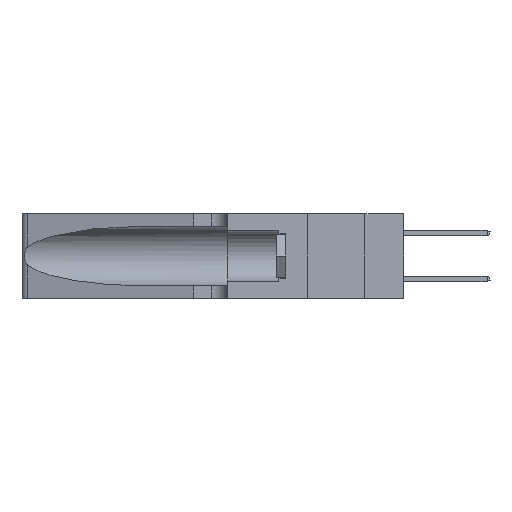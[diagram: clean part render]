
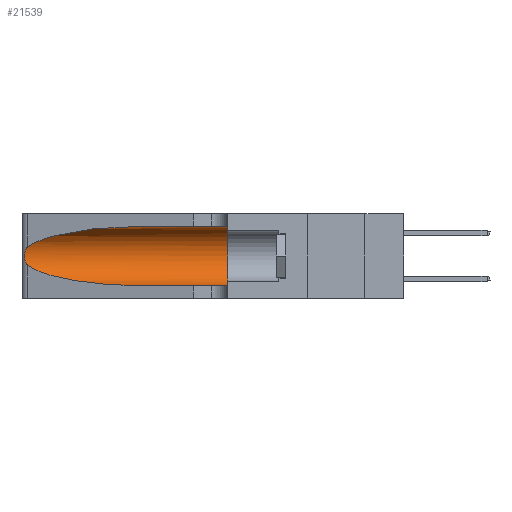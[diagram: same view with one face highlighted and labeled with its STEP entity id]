
A CAD part, left-side view. The second image highlights one B-rep face of the part: STEP entity #21539.
In plain terms, the highlighted cylindrical face has radius 3.308 mm (diameter 6.617 mm), a partial arc.
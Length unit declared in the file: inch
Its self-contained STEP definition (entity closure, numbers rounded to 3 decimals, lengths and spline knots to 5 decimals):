
#81 = ORIENTED_EDGE ( 'NONE', *, *, #700, .T. ) ;
#439 = ORIENTED_EDGE ( 'NONE', *, *, #10689, .T. ) ;
#695 =( BOUNDED_CURVE ( )  B_SPLINE_CURVE ( 3, ( #6078, #23244, #13934, #2161 ),
 .UNSPECIFIED., .F., .T. ) 
 B_SPLINE_CURVE_WITH_KNOTS ( ( 4, 4 ),
 ( 1.5708, 2.84003 ),
 .UNSPECIFIED. ) 
 CURVE ( )  GEOMETRIC_REPRESENTATION_ITEM ( )  RATIONAL_B_SPLINE_CURVE ( ( 1., 0.87, 0.87, 1. ) ) 
 REPRESENTATION_ITEM ( '' )  );
#700 = EDGE_CURVE ( 'NONE', #11478, #8818, #3081, .T. ) ;
#931 = CARTESIAN_POINT ( 'NONE',  ( 0.2373, 1.15595, 0.08982 ) ) ;
#1391 = CARTESIAN_POINT ( 'NONE',  ( 0.25854, 1.2359, 0.20912 ) ) ;
#1404 = ORIENTED_EDGE ( 'NONE', *, *, #21447, .T. ) ;
#1518 = VECTOR ( 'NONE', #3836, 39.37008 ) ;
#1533 = EDGE_CURVE ( 'NONE', #9029, #22695, #22541, .T. ) ;
#2071 = CARTESIAN_POINT ( 'NONE',  ( 0.25487, 1.22718, 0.14631 ) ) ;
#2156 = LINE ( 'NONE', #13624, #1518 ) ;
#2161 = CARTESIAN_POINT ( 'NONE',  ( 0.25487, 1.22718, 0.22369 ) ) ;
#2755 = CARTESIAN_POINT ( 'NONE',  ( 0.1305, 0.72297, 0.31525 ) ) ;
#2770 = VERTEX_POINT ( 'NONE', #15442 ) ;
#3007 = CARTESIAN_POINT ( 'NONE',  ( 0.26075, 1.23896, 0.178 ) ) ;
#3081 = B_SPLINE_CURVE_WITH_KNOTS ( 'NONE', 3,
 ( #7250, #7280, #14345, #20012, #1391, #10024, #15312, #3007, #6337, #12441, #22207, #12812, #7713, #16793 ),
 .UNSPECIFIED., .F., .F.,
 ( 4, 2, 2, 2, 2, 2, 4 ),
 ( 0., 0.00027, 0.00053, 0.00107, 0.0016, 0.00187, 0.00214 ),
 .UNSPECIFIED. ) ;
#3637 = AXIS2_PLACEMENT_3D ( 'NONE', #17673, #8112, #10079 ) ;
#3836 = DIRECTION ( 'NONE',  ( 0., -1., 0. ) ) ;
#3906 = CARTESIAN_POINT ( 'NONE',  ( 0.1305, 1.61858, 0.31525 ) ) ;
#4467 = CARTESIAN_POINT ( 'NONE',  ( 0.25487, 1.22718, 0.22369 ) ) ;
#4722 = ORIENTED_EDGE ( 'NONE', *, *, #1533, .F. ) ;
#5154 = ORIENTED_EDGE ( 'NONE', *, *, #22041, .F. ) ;
#6078 = CARTESIAN_POINT ( 'NONE',  ( 0.1305, 0.72297, 0.31525 ) ) ;
#6337 = CARTESIAN_POINT ( 'NONE',  ( 0.26017, 1.23833, 0.17102 ) ) ;
#6786 = ORIENTED_EDGE ( 'NONE', *, *, #15972, .T. ) ;
#7250 = CARTESIAN_POINT ( 'NONE',  ( 0.25487, 1.22718, 0.22369 ) ) ;
#7280 = CARTESIAN_POINT ( 'NONE',  ( 0.25555, 1.22994, 0.2215 ) ) ;
#7713 = CARTESIAN_POINT ( 'NONE',  ( 0.25555, 1.22993, 0.14849 ) ) ;
#7748 = CARTESIAN_POINT ( 'NONE',  ( 0.1305, 0.35, 0.185 ) ) ;
#8112 = DIRECTION ( 'NONE',  ( 0., -1., 0. ) ) ;
#8818 = VERTEX_POINT ( 'NONE', #2071 ) ;
#8952 = CARTESIAN_POINT ( 'NONE',  ( 0.1305, 0.72297, 0.05475 ) ) ;
#9029 = VERTEX_POINT ( 'NONE', #2755 ) ;
#9606 = FACE_OUTER_BOUND ( 'NONE', #15611, .T. ) ;
#9713 = DIRECTION ( 'NONE',  ( 0., 0., 1. ) ) ;
#10024 = CARTESIAN_POINT ( 'NONE',  ( 0.26018, 1.23835, 0.19895 ) ) ;
#10077 =( BOUNDED_CURVE ( )  B_SPLINE_CURVE ( 3, ( #18459, #931, #20355, #8952 ),
 .UNSPECIFIED., .F., .T. ) 
 B_SPLINE_CURVE_WITH_KNOTS ( ( 4, 4 ),
 ( 3.44316, 4.71239 ),
 .UNSPECIFIED. ) 
 CURVE ( )  GEOMETRIC_REPRESENTATION_ITEM ( )  RATIONAL_B_SPLINE_CURVE ( ( 1., 0.87, 0.87, 1. ) ) 
 REPRESENTATION_ITEM ( '' )  );
#10079 = DIRECTION ( 'NONE',  ( 0., 0., -1. ) ) ;
#10689 = EDGE_CURVE ( 'NONE', #9029, #11478, #695, .T. ) ;
#11099 = CIRCLE ( 'NONE', #17470, 0.13025 ) ;
#11478 = VERTEX_POINT ( 'NONE', #4467 ) ;
#12441 = CARTESIAN_POINT ( 'NONE',  ( 0.25856, 1.23593, 0.16098 ) ) ;
#12545 = VECTOR ( 'NONE', #21756, 39.37008 ) ;
#12558 = VERTEX_POINT ( 'NONE', #13332 ) ;
#12812 = CARTESIAN_POINT ( 'NONE',  ( 0.25639, 1.23186, 0.15144 ) ) ;
#13332 = CARTESIAN_POINT ( 'NONE',  ( 0.1305, 0.72297, 0.05475 ) ) ;
#13624 = CARTESIAN_POINT ( 'NONE',  ( 0.1305, 1.61858, 0.05475 ) ) ;
#13934 = CARTESIAN_POINT ( 'NONE',  ( 0.2373, 1.15595, 0.28018 ) ) ;
#14345 = CARTESIAN_POINT ( 'NONE',  ( 0.25639, 1.23184, 0.21858 ) ) ;
#15312 = CARTESIAN_POINT ( 'NONE',  ( 0.26075, 1.23896, 0.19203 ) ) ;
#15442 = CARTESIAN_POINT ( 'NONE',  ( 0.1305, 0.35, 0.05475 ) ) ;
#15611 = EDGE_LOOP ( 'NONE', ( #439, #81, #6786, #1404, #5154, #4722 ) ) ;
#15972 = EDGE_CURVE ( 'NONE', #8818, #12558, #10077, .T. ) ;
#16793 = CARTESIAN_POINT ( 'NONE',  ( 0.25487, 1.22718, 0.14631 ) ) ;
#17200 = CARTESIAN_POINT ( 'NONE',  ( 0.1305, 0.35, 0.31525 ) ) ;
#17470 = AXIS2_PLACEMENT_3D ( 'NONE', #7748, #21071, #9713 ) ;
#17673 = CARTESIAN_POINT ( 'NONE',  ( 0.1305, 1.61858, 0.185 ) ) ;
#18459 = CARTESIAN_POINT ( 'NONE',  ( 0.25487, 1.22718, 0.14631 ) ) ;
#20012 = CARTESIAN_POINT ( 'NONE',  ( 0.25787, 1.23484, 0.2124 ) ) ;
#20355 = CARTESIAN_POINT ( 'NONE',  ( 0.18966, 0.96281, 0.05475 ) ) ;
#21071 = DIRECTION ( 'NONE',  ( 0., 1., 0. ) ) ;
#21447 = EDGE_CURVE ( 'NONE', #12558, #2770, #2156, .T. ) ;
#21539 = ADVANCED_FACE ( 'NONE', ( #9606 ), #23483, .F. ) ;
#21756 = DIRECTION ( 'NONE',  ( 0., -1., 0. ) ) ;
#22041 = EDGE_CURVE ( 'NONE', #22695, #2770, #11099, .T. ) ;
#22207 = CARTESIAN_POINT ( 'NONE',  ( 0.25789, 1.23486, 0.15765 ) ) ;
#22541 = LINE ( 'NONE', #3906, #12545 ) ;
#22695 = VERTEX_POINT ( 'NONE', #17200 ) ;
#23244 = CARTESIAN_POINT ( 'NONE',  ( 0.18966, 0.96281, 0.31525 ) ) ;
#23483 = CYLINDRICAL_SURFACE ( 'NONE', #3637, 0.13025 ) ;
